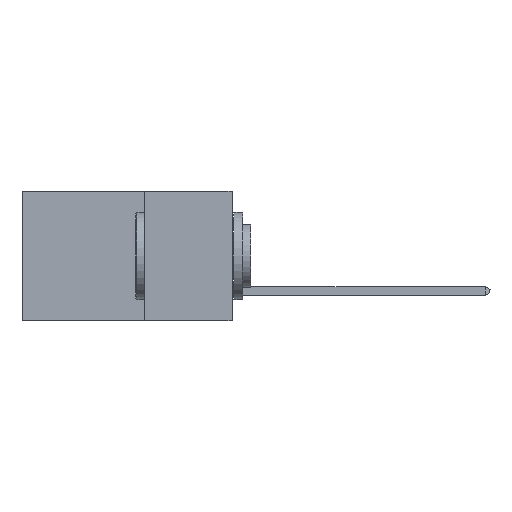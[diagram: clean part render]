
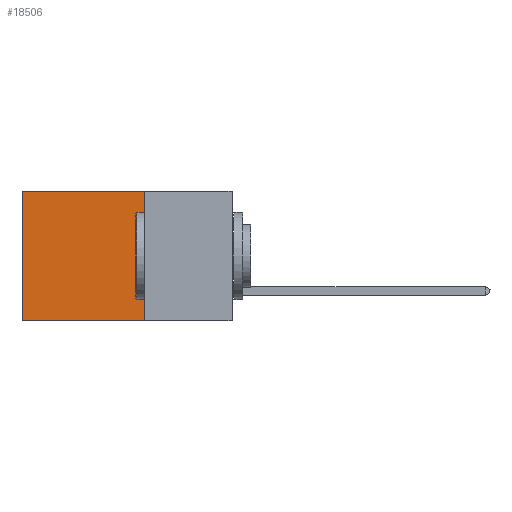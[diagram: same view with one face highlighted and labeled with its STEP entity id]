
A CAD part, left-side view. The second image highlights one B-rep face of the part: STEP entity #18506.
In plain terms, the highlighted planar face has unit normal (-1, 0, 0).
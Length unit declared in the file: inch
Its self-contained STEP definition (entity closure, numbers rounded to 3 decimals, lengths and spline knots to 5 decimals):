
#601 = VECTOR ( 'NONE', #3263, 39.37008 ) ;
#896 = VECTOR ( 'NONE', #19059, 39.37008 ) ;
#905 = ORIENTED_EDGE ( 'NONE', *, *, #3892, .T. ) ;
#1774 = VERTEX_POINT ( 'NONE', #22695 ) ;
#1802 = DIRECTION ( 'NONE',  ( 0., 0., -1. ) ) ;
#1886 = VECTOR ( 'NONE', #11447, 39.37008 ) ;
#3263 = DIRECTION ( 'NONE',  ( 0., 1., 0. ) ) ;
#3892 = EDGE_CURVE ( 'NONE', #25398, #5082, #14275, .T. ) ;
#5082 = VERTEX_POINT ( 'NONE', #17376 ) ;
#11447 = DIRECTION ( 'NONE',  ( 0., 0., -1. ) ) ;
#13498 = CARTESIAN_POINT ( 'NONE',  ( 0.2875, 0.25, 0. ) ) ;
#14275 = LINE ( 'NONE', #33924, #601 ) ;
#14417 = ORIENTED_EDGE ( 'NONE', *, *, #19592, .T. ) ;
#15125 = EDGE_CURVE ( 'NONE', #25398, #20591, #33701, .T. ) ;
#17376 = CARTESIAN_POINT ( 'NONE',  ( 0.2875, 0.6, 0. ) ) ;
#17589 = LINE ( 'NONE', #20321, #1886 ) ;
#18464 = FACE_OUTER_BOUND ( 'NONE', #30488, .T. ) ;
#18506 = ADVANCED_FACE ( 'NONE', ( #18464 ), #26914, .F. ) ;
#19059 = DIRECTION ( 'NONE',  ( 0., 1., 0. ) ) ;
#19399 = AXIS2_PLACEMENT_3D ( 'NONE', #13498, #30141, #25035 ) ;
#19434 = CARTESIAN_POINT ( 'NONE',  ( 0.2875, 0.25, -0.37 ) ) ;
#19524 = CARTESIAN_POINT ( 'NONE',  ( 0.2875, 0.25, -0.37 ) ) ;
#19592 = EDGE_CURVE ( 'NONE', #5082, #1774, #17589, .T. ) ;
#20169 = ORIENTED_EDGE ( 'NONE', *, *, #15125, .F. ) ;
#20321 = CARTESIAN_POINT ( 'NONE',  ( 0.2875, 0.6, 0. ) ) ;
#20591 = VERTEX_POINT ( 'NONE', #19434 ) ;
#22695 = CARTESIAN_POINT ( 'NONE',  ( 0.2875, 0.6, -0.37 ) ) ;
#23069 = CARTESIAN_POINT ( 'NONE',  ( 0.2875, 0.25, 0. ) ) ;
#24313 = VECTOR ( 'NONE', #1802, 39.37008 ) ;
#25035 = DIRECTION ( 'NONE',  ( 0., 0., -1. ) ) ;
#25398 = VERTEX_POINT ( 'NONE', #23069 ) ;
#26109 = EDGE_CURVE ( 'NONE', #20591, #1774, #28053, .T. ) ;
#26914 = PLANE ( 'NONE',  #19399 ) ;
#28053 = LINE ( 'NONE', #19524, #896 ) ;
#30141 = DIRECTION ( 'NONE',  ( 1., 0., 0. ) ) ;
#30488 = EDGE_LOOP ( 'NONE', ( #14417, #32113, #20169, #905 ) ) ;
#32113 = ORIENTED_EDGE ( 'NONE', *, *, #26109, .F. ) ;
#33701 = LINE ( 'NONE', #33995, #24313 ) ;
#33924 = CARTESIAN_POINT ( 'NONE',  ( 0.2875, 0.25, 0. ) ) ;
#33995 = CARTESIAN_POINT ( 'NONE',  ( 0.2875, 0.25, 0. ) ) ;
